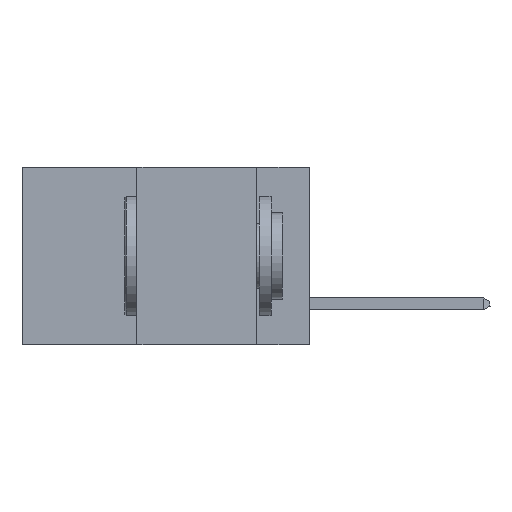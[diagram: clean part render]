
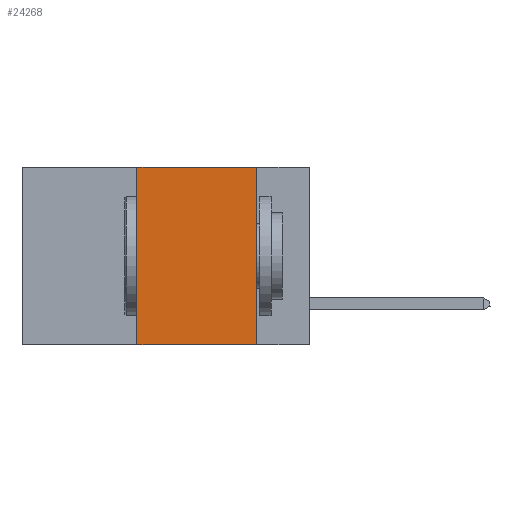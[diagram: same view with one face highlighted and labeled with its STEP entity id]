
A CAD part, left-side view. The second image highlights one B-rep face of the part: STEP entity #24268.
In plain terms, the highlighted planar face has unit normal (-1, 0, 0).
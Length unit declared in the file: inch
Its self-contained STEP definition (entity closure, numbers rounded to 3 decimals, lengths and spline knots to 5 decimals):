
#511 = ORIENTED_EDGE ( 'NONE', *, *, #24298, .F. ) ;
#932 = LINE ( 'NONE', #27819, #28092 ) ;
#1851 = EDGE_CURVE ( 'NONE', #16458, #30863, #932, .T. ) ;
#4893 = DIRECTION ( 'NONE',  ( 0., 0., -1. ) ) ;
#5880 = DIRECTION ( 'NONE',  ( 0., -1., 0. ) ) ;
#6972 = CARTESIAN_POINT ( 'NONE',  ( 0., 0.11, 0. ) ) ;
#7903 = AXIS2_PLACEMENT_3D ( 'NONE', #9022, #14162, #13842 ) ;
#8178 = EDGE_LOOP ( 'NONE', ( #18921, #22021, #511, #31105 ) ) ;
#8294 = EDGE_CURVE ( 'NONE', #20235, #11232, #15547, .T. ) ;
#9022 = CARTESIAN_POINT ( 'NONE',  ( 0., 0.6, 0. ) ) ;
#9177 = VECTOR ( 'NONE', #5880, 39.37008 ) ;
#9241 = PLANE ( 'NONE',  #7903 ) ;
#11232 = VERTEX_POINT ( 'NONE', #6972 ) ;
#11950 = LINE ( 'NONE', #28642, #21753 ) ;
#13842 = DIRECTION ( 'NONE',  ( 0., 0., -1. ) ) ;
#14162 = DIRECTION ( 'NONE',  ( 1., 0., 0. ) ) ;
#14253 = CARTESIAN_POINT ( 'NONE',  ( 0., 0.11, 0. ) ) ;
#14714 = VECTOR ( 'NONE', #4893, 39.37008 ) ;
#15547 = LINE ( 'NONE', #20002, #9177 ) ;
#16087 = EDGE_CURVE ( 'NONE', #11232, #30863, #21895, .T. ) ;
#16352 = CARTESIAN_POINT ( 'NONE',  ( 0., 0.11, -0.37 ) ) ;
#16458 = VERTEX_POINT ( 'NONE', #22052 ) ;
#17594 = FACE_OUTER_BOUND ( 'NONE', #8178, .T. ) ;
#18921 = ORIENTED_EDGE ( 'NONE', *, *, #16087, .F. ) ;
#20002 = CARTESIAN_POINT ( 'NONE',  ( 0., 0.6, 0. ) ) ;
#20235 = VERTEX_POINT ( 'NONE', #22239 ) ;
#21251 = DIRECTION ( 'NONE',  ( 0., 0., 1. ) ) ;
#21753 = VECTOR ( 'NONE', #21251, 39.37008 ) ;
#21895 = LINE ( 'NONE', #14253, #14714 ) ;
#22021 = ORIENTED_EDGE ( 'NONE', *, *, #8294, .F. ) ;
#22052 = CARTESIAN_POINT ( 'NONE',  ( 0., 0.36, -0.37 ) ) ;
#22239 = CARTESIAN_POINT ( 'NONE',  ( 0., 0.36, 0. ) ) ;
#24268 = ADVANCED_FACE ( 'NONE', ( #17594 ), #9241, .F. ) ;
#24298 = EDGE_CURVE ( 'NONE', #16458, #20235, #11950, .T. ) ;
#27819 = CARTESIAN_POINT ( 'NONE',  ( 0., 0.6, -0.37 ) ) ;
#28092 = VECTOR ( 'NONE', #31052, 39.37008 ) ;
#28642 = CARTESIAN_POINT ( 'NONE',  ( 0., 0.36, 0. ) ) ;
#30863 = VERTEX_POINT ( 'NONE', #16352 ) ;
#31052 = DIRECTION ( 'NONE',  ( 0., -1., 0. ) ) ;
#31105 = ORIENTED_EDGE ( 'NONE', *, *, #1851, .T. ) ;
